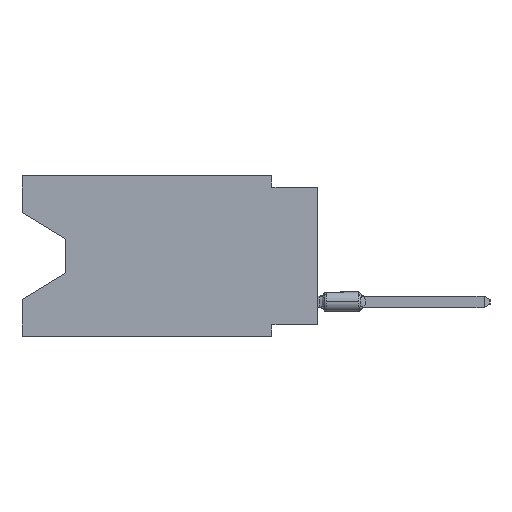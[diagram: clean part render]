
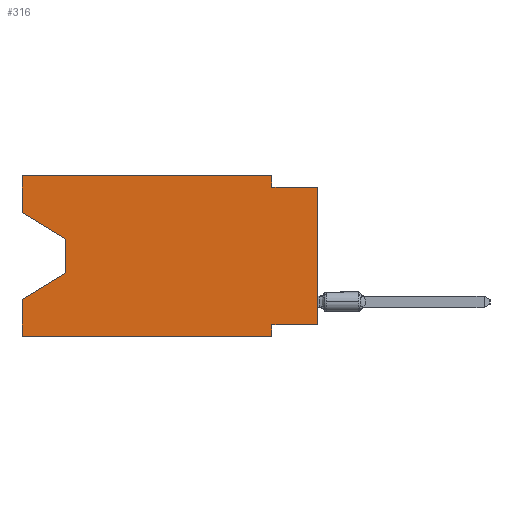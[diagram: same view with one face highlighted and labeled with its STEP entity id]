
A CAD part, left-side view. The second image highlights one B-rep face of the part: STEP entity #316.
In plain terms, the highlighted planar face has unit normal (-1, 0, 0).
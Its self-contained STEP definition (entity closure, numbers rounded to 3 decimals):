
#316 = ADVANCED_FACE ( 'NONE', ( #2772 ), #3285, .F. ) ;
#998 = VECTOR ( 'NONE', #4854, 1000. ) ;
#1560 = VERTEX_POINT ( 'NONE', #25632 ) ;
#2447 = LINE ( 'NONE', #50711, #11732 ) ;
#2703 = LINE ( 'NONE', #18033, #8115 ) ;
#2772 = FACE_OUTER_BOUND ( 'NONE', #33774, .T. ) ;
#3285 = PLANE ( 'NONE',  #31392 ) ;
#3335 = CARTESIAN_POINT ( 'NONE',  ( 0., 16.383, -2.038 ) ) ;
#3735 = DIRECTION ( 'NONE',  ( 0., 0., -1. ) ) ;
#4107 = LINE ( 'NONE', #16256, #23577 ) ;
#4150 = VECTOR ( 'NONE', #20365, 1000. ) ;
#4845 = ORIENTED_EDGE ( 'NONE', *, *, #27927, .F. ) ;
#4854 = DIRECTION ( 'NONE',  ( 0., 1., 0. ) ) ;
#5371 = ORIENTED_EDGE ( 'NONE', *, *, #17051, .T. ) ;
#6298 = VERTEX_POINT ( 'NONE', #15054 ) ;
#6868 = ORIENTED_EDGE ( 'NONE', *, *, #46985, .F. ) ;
#7125 = CARTESIAN_POINT ( 'NONE',  ( 0., 16.383, -2.038 ) ) ;
#7224 = ORIENTED_EDGE ( 'NONE', *, *, #38954, .T. ) ;
#7507 = ORIENTED_EDGE ( 'NONE', *, *, #30760, .T. ) ;
#7820 = VERTEX_POINT ( 'NONE', #51880 ) ;
#8115 = VECTOR ( 'NONE', #47009, 1000. ) ;
#8534 = VECTOR ( 'NONE', #43360, 1000. ) ;
#8912 = CARTESIAN_POINT ( 'NONE',  ( 0., 2.54, -0.635 ) ) ;
#10117 = EDGE_CURVE ( 'NONE', #1560, #23470, #27778, .T. ) ;
#11732 = VECTOR ( 'NONE', #20070, 1000. ) ;
#12936 = VECTOR ( 'NONE', #13385, 1000. ) ;
#13385 = DIRECTION ( 'NONE',  ( 0., 0., -1. ) ) ;
#14901 = CARTESIAN_POINT ( 'NONE',  ( 0., 16.383, 0. ) ) ;
#15054 = CARTESIAN_POINT ( 'NONE',  ( 0., 13.97, -3.505 ) ) ;
#15395 = VECTOR ( 'NONE', #23222, 1000. ) ;
#16256 = CARTESIAN_POINT ( 'NONE',  ( 0., 13.97, -5.385 ) ) ;
#17051 = EDGE_CURVE ( 'NONE', #26513, #6298, #26951, .T. ) ;
#17253 = CARTESIAN_POINT ( 'NONE',  ( 0., 16.383, -6.852 ) ) ;
#18033 = CARTESIAN_POINT ( 'NONE',  ( 0., 16.383, 0. ) ) ;
#18228 = VERTEX_POINT ( 'NONE', #17253 ) ;
#18541 = VECTOR ( 'NONE', #35751, 1000. ) ;
#18768 = EDGE_CURVE ( 'NONE', #26513, #30805, #31977, .T. ) ;
#19346 = CARTESIAN_POINT ( 'NONE',  ( 0., 0., -8.255 ) ) ;
#19431 = CARTESIAN_POINT ( 'NONE',  ( 0., 0., -0.635 ) ) ;
#20070 = DIRECTION ( 'NONE',  ( 0., 0., -1. ) ) ;
#20119 = ORIENTED_EDGE ( 'NONE', *, *, #18768, .F. ) ;
#20365 = DIRECTION ( 'NONE',  ( 0., 0., 1. ) ) ;
#23222 = DIRECTION ( 'NONE',  ( 0., -0.855, -0.519 ) ) ;
#23470 = VERTEX_POINT ( 'NONE', #47857 ) ;
#23577 = VECTOR ( 'NONE', #51833, 1000. ) ;
#23813 = CARTESIAN_POINT ( 'NONE',  ( 0., 2.54, -8.89 ) ) ;
#24203 = LINE ( 'NONE', #48990, #47162 ) ;
#24297 = CARTESIAN_POINT ( 'NONE',  ( 0., 16.383, 0. ) ) ;
#24905 = LINE ( 'NONE', #41003, #998 ) ;
#25632 = CARTESIAN_POINT ( 'NONE',  ( 0., 2.54, -8.255 ) ) ;
#25783 = CARTESIAN_POINT ( 'NONE',  ( 0., 2.54, 0. ) ) ;
#26513 = VERTEX_POINT ( 'NONE', #3335 ) ;
#26530 = LINE ( 'NONE', #27302, #8534 ) ;
#26951 = LINE ( 'NONE', #7125, #15395 ) ;
#27060 = VERTEX_POINT ( 'NONE', #29129 ) ;
#27302 = CARTESIAN_POINT ( 'NONE',  ( 0., 16.383, 0. ) ) ;
#27778 = LINE ( 'NONE', #23813, #41687 ) ;
#27927 = EDGE_CURVE ( 'NONE', #30805, #7820, #2703, .T. ) ;
#28639 = VERTEX_POINT ( 'NONE', #19431 ) ;
#29129 = CARTESIAN_POINT ( 'NONE',  ( 0., 13.97, -5.385 ) ) ;
#30289 = ORIENTED_EDGE ( 'NONE', *, *, #51930, .F. ) ;
#30725 = VERTEX_POINT ( 'NONE', #51464 ) ;
#30760 = EDGE_CURVE ( 'NONE', #6298, #27060, #2447, .T. ) ;
#30805 = VERTEX_POINT ( 'NONE', #24297 ) ;
#31010 = DIRECTION ( 'NONE',  ( 0., 0., -1. ) ) ;
#31392 = AXIS2_PLACEMENT_3D ( 'NONE', #14901, #31519, #31010 ) ;
#31519 = DIRECTION ( 'NONE',  ( 1., 0., 0. ) ) ;
#31977 = LINE ( 'NONE', #48058, #4150 ) ;
#33122 = CARTESIAN_POINT ( 'NONE',  ( 0., 16.383, -8.89 ) ) ;
#33416 = LINE ( 'NONE', #25783, #12936 ) ;
#33774 = EDGE_LOOP ( 'NONE', ( #5371, #7507, #43525, #6868, #7224, #41940, #34001, #39460, #30289, #51603, #4845, #20119 ) ) ;
#33965 = VECTOR ( 'NONE', #44174, 1000. ) ;
#34001 = ORIENTED_EDGE ( 'NONE', *, *, #49536, .F. ) ;
#35566 = EDGE_CURVE ( 'NONE', #27060, #18228, #4107, .T. ) ;
#35751 = DIRECTION ( 'NONE',  ( 0., 0., 1. ) ) ;
#36156 = EDGE_CURVE ( 'NONE', #38168, #28639, #52096, .T. ) ;
#37582 = VERTEX_POINT ( 'NONE', #8912 ) ;
#38168 = VERTEX_POINT ( 'NONE', #19346 ) ;
#38954 = EDGE_CURVE ( 'NONE', #30725, #23470, #45239, .T. ) ;
#39460 = ORIENTED_EDGE ( 'NONE', *, *, #36156, .T. ) ;
#41003 = CARTESIAN_POINT ( 'NONE',  ( 0., 0., -8.255 ) ) ;
#41687 = VECTOR ( 'NONE', #3735, 1000. ) ;
#41940 = ORIENTED_EDGE ( 'NONE', *, *, #10117, .F. ) ;
#43360 = DIRECTION ( 'NONE',  ( 0., 0., 1. ) ) ;
#43525 = ORIENTED_EDGE ( 'NONE', *, *, #35566, .T. ) ;
#44174 = DIRECTION ( 'NONE',  ( 0., -1., 0. ) ) ;
#44508 = DIRECTION ( 'NONE',  ( 0., -1., 0. ) ) ;
#45239 = LINE ( 'NONE', #33122, #33965 ) ;
#46985 = EDGE_CURVE ( 'NONE', #30725, #18228, #26530, .T. ) ;
#47009 = DIRECTION ( 'NONE',  ( 0., -1., 0. ) ) ;
#47162 = VECTOR ( 'NONE', #44508, 1000. ) ;
#47857 = CARTESIAN_POINT ( 'NONE',  ( 0., 2.54, -8.89 ) ) ;
#48058 = CARTESIAN_POINT ( 'NONE',  ( 0., 16.383, 0. ) ) ;
#48155 = CARTESIAN_POINT ( 'NONE',  ( 0., 0., 0. ) ) ;
#48990 = CARTESIAN_POINT ( 'NONE',  ( 0., 0., -0.635 ) ) ;
#49536 = EDGE_CURVE ( 'NONE', #38168, #1560, #24905, .T. ) ;
#50711 = CARTESIAN_POINT ( 'NONE',  ( 0., 13.97, -3.505 ) ) ;
#50790 = EDGE_CURVE ( 'NONE', #7820, #37582, #33416, .T. ) ;
#51464 = CARTESIAN_POINT ( 'NONE',  ( 0., 16.383, -8.89 ) ) ;
#51603 = ORIENTED_EDGE ( 'NONE', *, *, #50790, .F. ) ;
#51833 = DIRECTION ( 'NONE',  ( 0., 0.855, -0.519 ) ) ;
#51880 = CARTESIAN_POINT ( 'NONE',  ( 0., 2.54, 0. ) ) ;
#51930 = EDGE_CURVE ( 'NONE', #37582, #28639, #24203, .T. ) ;
#52096 = LINE ( 'NONE', #48155, #18541 ) ;
